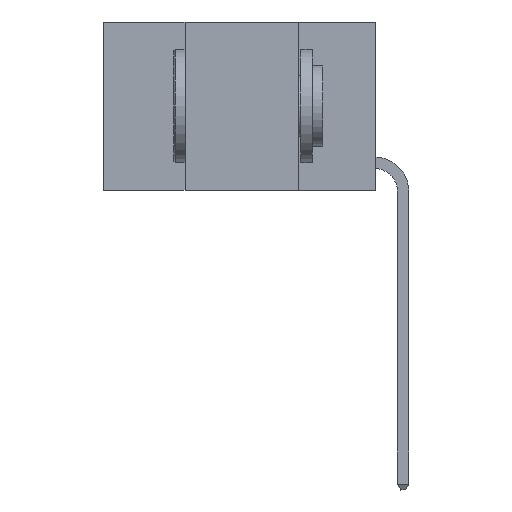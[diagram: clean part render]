
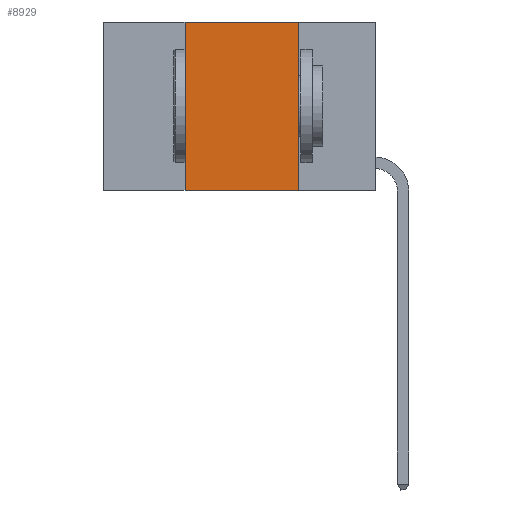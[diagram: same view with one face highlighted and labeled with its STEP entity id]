
A CAD part, left-side view. The second image highlights one B-rep face of the part: STEP entity #8929.
In plain terms, the highlighted planar face has unit normal (-1, 0, 0).
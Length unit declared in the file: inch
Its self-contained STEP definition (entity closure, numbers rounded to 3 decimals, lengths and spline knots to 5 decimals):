
#242 = CARTESIAN_POINT ( 'NONE',  ( 0., 0.17, 0. ) ) ;
#579 = ORIENTED_EDGE ( 'NONE', *, *, #10980, .F. ) ;
#774 = AXIS2_PLACEMENT_3D ( 'NONE', #14361, #6236, #17144 ) ;
#810 = FACE_OUTER_BOUND ( 'NONE', #1030, .T. ) ;
#855 = EDGE_CURVE ( 'NONE', #7925, #9645, #15320, .T. ) ;
#1030 = EDGE_LOOP ( 'NONE', ( #579, #5023, #6012, #13861 ) ) ;
#1575 = VECTOR ( 'NONE', #16554, 39.37008 ) ;
#1670 = CARTESIAN_POINT ( 'NONE',  ( 0., 0.42, 0. ) ) ;
#3109 = LINE ( 'NONE', #242, #9059 ) ;
#4308 = LINE ( 'NONE', #13566, #1575 ) ;
#4384 = DIRECTION ( 'NONE',  ( 0., -1., 0. ) ) ;
#5023 = ORIENTED_EDGE ( 'NONE', *, *, #15705, .F. ) ;
#5597 = EDGE_CURVE ( 'NONE', #7925, #6815, #4308, .T. ) ;
#5640 = CARTESIAN_POINT ( 'NONE',  ( 0., 0.6, 0. ) ) ;
#6012 = ORIENTED_EDGE ( 'NONE', *, *, #855, .F. ) ;
#6236 = DIRECTION ( 'NONE',  ( 1., 0., 0. ) ) ;
#6815 = VERTEX_POINT ( 'NONE', #11883 ) ;
#7925 = VERTEX_POINT ( 'NONE', #9671 ) ;
#8749 = VECTOR ( 'NONE', #13954, 39.37008 ) ;
#8929 = ADVANCED_FACE ( 'NONE', ( #810 ), #12822, .F. ) ;
#9059 = VECTOR ( 'NONE', #12349, 39.37008 ) ;
#9645 = VERTEX_POINT ( 'NONE', #1670 ) ;
#9671 = CARTESIAN_POINT ( 'NONE',  ( 0., 0.42, -0.37 ) ) ;
#10007 = CARTESIAN_POINT ( 'NONE',  ( 0., 0.42, 0. ) ) ;
#10980 = EDGE_CURVE ( 'NONE', #14877, #6815, #3109, .T. ) ;
#11034 = CARTESIAN_POINT ( 'NONE',  ( 0., 0.17, 0. ) ) ;
#11883 = CARTESIAN_POINT ( 'NONE',  ( 0., 0.17, -0.37 ) ) ;
#12308 = LINE ( 'NONE', #5640, #16874 ) ;
#12349 = DIRECTION ( 'NONE',  ( 0., 0., -1. ) ) ;
#12822 = PLANE ( 'NONE',  #774 ) ;
#13566 = CARTESIAN_POINT ( 'NONE',  ( 0., 0.6, -0.37 ) ) ;
#13861 = ORIENTED_EDGE ( 'NONE', *, *, #5597, .T. ) ;
#13954 = DIRECTION ( 'NONE',  ( 0., 0., 1. ) ) ;
#14361 = CARTESIAN_POINT ( 'NONE',  ( 0., 0.6, 0. ) ) ;
#14877 = VERTEX_POINT ( 'NONE', #11034 ) ;
#15320 = LINE ( 'NONE', #10007, #8749 ) ;
#15705 = EDGE_CURVE ( 'NONE', #9645, #14877, #12308, .T. ) ;
#16554 = DIRECTION ( 'NONE',  ( 0., -1., 0. ) ) ;
#16874 = VECTOR ( 'NONE', #4384, 39.37008 ) ;
#17144 = DIRECTION ( 'NONE',  ( 0., 0., -1. ) ) ;
